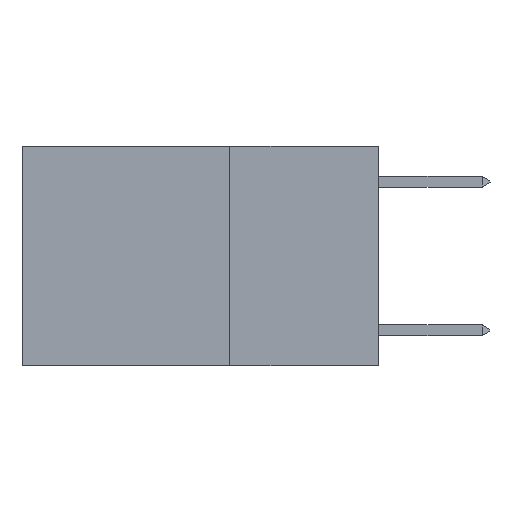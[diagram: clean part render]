
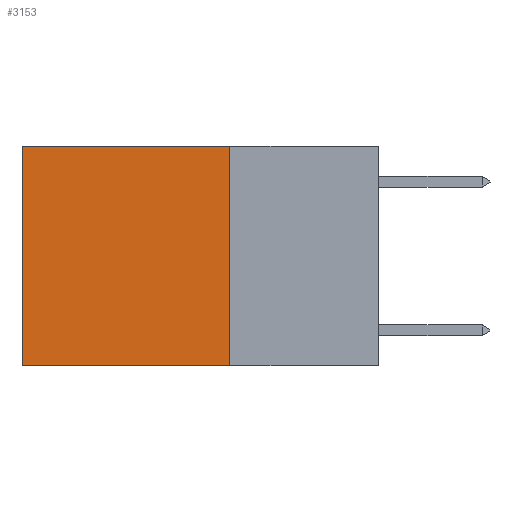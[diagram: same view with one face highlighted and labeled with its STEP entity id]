
A CAD part, left-side view. The second image highlights one B-rep face of the part: STEP entity #3153.
In plain terms, the highlighted planar face has unit normal (-1, 0, 0).
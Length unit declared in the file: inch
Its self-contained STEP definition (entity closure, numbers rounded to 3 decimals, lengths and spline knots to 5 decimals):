
#615 = ORIENTED_EDGE ( 'NONE', *, *, #10440, .T. ) ;
#756 = CARTESIAN_POINT ( 'NONE',  ( 0.2625, 0.25, -0.37 ) ) ;
#879 = ORIENTED_EDGE ( 'NONE', *, *, #3037, .F. ) ;
#1033 = DIRECTION ( 'NONE',  ( 0., 1., 0. ) ) ;
#1882 = FACE_OUTER_BOUND ( 'NONE', #14946, .T. ) ;
#2996 = DIRECTION ( 'NONE',  ( 0., 0., -1. ) ) ;
#3037 = EDGE_CURVE ( 'NONE', #18962, #13972, #15615, .T. ) ;
#3153 = ADVANCED_FACE ( 'NONE', ( #1882 ), #18114, .F. ) ;
#3305 = VECTOR ( 'NONE', #1033, 39.37008 ) ;
#4212 = VECTOR ( 'NONE', #2996, 39.37008 ) ;
#5287 = LINE ( 'NONE', #8119, #4212 ) ;
#6764 = EDGE_CURVE ( 'NONE', #13972, #16207, #20944, .T. ) ;
#8119 = CARTESIAN_POINT ( 'NONE',  ( 0.2625, 0.6, 0. ) ) ;
#8346 = LINE ( 'NONE', #21162, #3305 ) ;
#9253 = DIRECTION ( 'NONE',  ( 0., 0., -1. ) ) ;
#10440 = EDGE_CURVE ( 'NONE', #18730, #16207, #5287, .T. ) ;
#11475 = CARTESIAN_POINT ( 'NONE',  ( 0.2625, 0.25, 0. ) ) ;
#12898 = VECTOR ( 'NONE', #18726, 39.37008 ) ;
#13189 = DIRECTION ( 'NONE',  ( 0., 0., -1. ) ) ;
#13972 = VERTEX_POINT ( 'NONE', #756 ) ;
#14946 = EDGE_LOOP ( 'NONE', ( #615, #15504, #879, #17698 ) ) ;
#15274 = AXIS2_PLACEMENT_3D ( 'NONE', #11475, #16572, #13189 ) ;
#15504 = ORIENTED_EDGE ( 'NONE', *, *, #6764, .F. ) ;
#15615 = LINE ( 'NONE', #15702, #18481 ) ;
#15702 = CARTESIAN_POINT ( 'NONE',  ( 0.2625, 0.25, 0. ) ) ;
#16207 = VERTEX_POINT ( 'NONE', #18969 ) ;
#16572 = DIRECTION ( 'NONE',  ( 1., 0., 0. ) ) ;
#17698 = ORIENTED_EDGE ( 'NONE', *, *, #18623, .T. ) ;
#18114 = PLANE ( 'NONE',  #15274 ) ;
#18428 = CARTESIAN_POINT ( 'NONE',  ( 0.2625, 0.25, 0. ) ) ;
#18481 = VECTOR ( 'NONE', #9253, 39.37008 ) ;
#18623 = EDGE_CURVE ( 'NONE', #18962, #18730, #8346, .T. ) ;
#18726 = DIRECTION ( 'NONE',  ( 0., 1., 0. ) ) ;
#18730 = VERTEX_POINT ( 'NONE', #19837 ) ;
#18873 = CARTESIAN_POINT ( 'NONE',  ( 0.2625, 0.25, -0.37 ) ) ;
#18962 = VERTEX_POINT ( 'NONE', #18428 ) ;
#18969 = CARTESIAN_POINT ( 'NONE',  ( 0.2625, 0.6, -0.37 ) ) ;
#19837 = CARTESIAN_POINT ( 'NONE',  ( 0.2625, 0.6, 0. ) ) ;
#20944 = LINE ( 'NONE', #18873, #12898 ) ;
#21162 = CARTESIAN_POINT ( 'NONE',  ( 0.2625, 0.25, 0. ) ) ;
